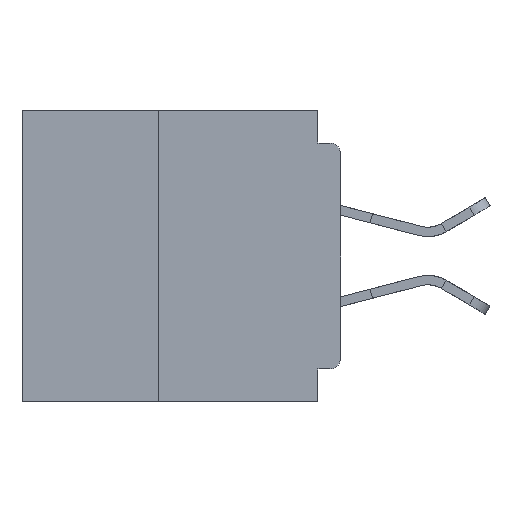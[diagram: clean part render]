
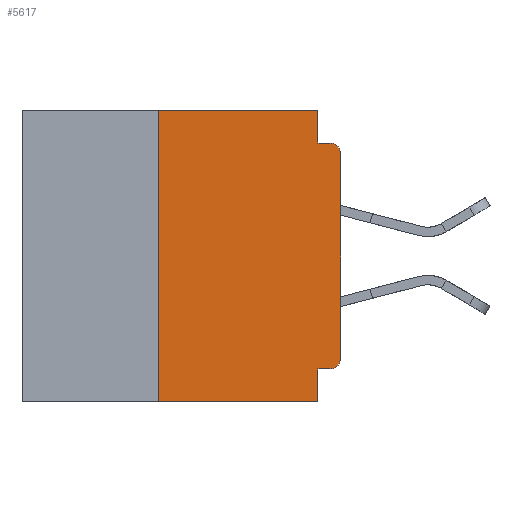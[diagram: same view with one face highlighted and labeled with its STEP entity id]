
A CAD part, left-side view. The second image highlights one B-rep face of the part: STEP entity #5617.
In plain terms, the highlighted planar face has unit normal (-1, 0, 0).
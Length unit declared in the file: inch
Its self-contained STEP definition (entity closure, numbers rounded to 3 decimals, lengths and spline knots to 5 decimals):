
#760 = EDGE_LOOP ( 'NONE', ( #19155, #7174, #18591, #26904, #25156, #31507, #24064, #19245, #5497, #3072 ) ) ;
#850 = DIRECTION ( 'NONE',  ( 0., -1., 0. ) ) ;
#874 = VECTOR ( 'NONE', #28364, 39.37008 ) ;
#1876 = CARTESIAN_POINT ( 'NONE',  ( 0., 0.031, -0.355 ) ) ;
#2531 = CIRCLE ( 'NONE', #13504, 0.015 ) ;
#3072 = ORIENTED_EDGE ( 'NONE', *, *, #12800, .T. ) ;
#3850 = LINE ( 'NONE', #40237, #29179 ) ;
#5197 = DIRECTION ( 'NONE',  ( -1., 0., 0. ) ) ;
#5497 = ORIENTED_EDGE ( 'NONE', *, *, #16973, .F. ) ;
#5546 = LINE ( 'NONE', #32542, #23152 ) ;
#5617 = ADVANCED_FACE ( 'NONE', ( #33555 ), #7293, .F. ) ;
#5638 = CARTESIAN_POINT ( 'NONE',  ( 0., 0., -0.34 ) ) ;
#6015 = VERTEX_POINT ( 'NONE', #8084 ) ;
#6121 = CARTESIAN_POINT ( 'NONE',  ( 0., 0.015, -0.34 ) ) ;
#6954 = CARTESIAN_POINT ( 'NONE',  ( 0., 0., 0. ) ) ;
#7174 = ORIENTED_EDGE ( 'NONE', *, *, #29271, .T. ) ;
#7293 = PLANE ( 'NONE',  #39121 ) ;
#8084 = CARTESIAN_POINT ( 'NONE',  ( 0., 0., -0.06 ) ) ;
#9132 = LINE ( 'NONE', #10199, #25701 ) ;
#9355 = CARTESIAN_POINT ( 'NONE',  ( 0., 0.031, -0.4 ) ) ;
#9437 = DIRECTION ( 'NONE',  ( 0., 0., -1. ) ) ;
#9480 = DIRECTION ( 'NONE',  ( 0., 0., -1. ) ) ;
#9642 = VERTEX_POINT ( 'NONE', #5638 ) ;
#10199 = CARTESIAN_POINT ( 'NONE',  ( 0., 0., -0.045 ) ) ;
#10797 = VERTEX_POINT ( 'NONE', #1876 ) ;
#11813 = VECTOR ( 'NONE', #39659, 39.37008 ) ;
#12800 = EDGE_CURVE ( 'NONE', #18607, #9642, #20574, .T. ) ;
#12972 = EDGE_CURVE ( 'NONE', #9642, #6015, #23135, .T. ) ;
#13504 = AXIS2_PLACEMENT_3D ( 'NONE', #25016, #5197, #28303 ) ;
#13541 = DIRECTION ( 'NONE',  ( 0., -1., 0. ) ) ;
#13967 = VECTOR ( 'NONE', #14955, 39.37008 ) ;
#14865 = VERTEX_POINT ( 'NONE', #29692 ) ;
#14955 = DIRECTION ( 'NONE',  ( 0., 1., 0. ) ) ;
#16574 = VERTEX_POINT ( 'NONE', #9355 ) ;
#16596 = CARTESIAN_POINT ( 'NONE',  ( 0., 0.031, -0.4 ) ) ;
#16973 = EDGE_CURVE ( 'NONE', #18607, #10797, #22765, .T. ) ;
#17788 = EDGE_CURVE ( 'NONE', #14865, #20665, #26785, .T. ) ;
#18015 = VECTOR ( 'NONE', #40280, 39.37008 ) ;
#18419 = CARTESIAN_POINT ( 'NONE',  ( 0., 0.437, -0.4 ) ) ;
#18591 = ORIENTED_EDGE ( 'NONE', *, *, #30137, .F. ) ;
#18607 = VERTEX_POINT ( 'NONE', #41528 ) ;
#19155 = ORIENTED_EDGE ( 'NONE', *, *, #12972, .T. ) ;
#19245 = ORIENTED_EDGE ( 'NONE', *, *, #34784, .F. ) ;
#20331 = EDGE_CURVE ( 'NONE', #20665, #31891, #3850, .T. ) ;
#20574 = CIRCLE ( 'NONE', #31055, 0.015 ) ;
#20590 = CARTESIAN_POINT ( 'NONE',  ( 0., 0.25, -0.4 ) ) ;
#20630 = LINE ( 'NONE', #16596, #11813 ) ;
#20636 = DIRECTION ( 'NONE',  ( 0., 0., -1. ) ) ;
#20665 = VERTEX_POINT ( 'NONE', #22701 ) ;
#22105 = VECTOR ( 'NONE', #26763, 39.37008 ) ;
#22701 = CARTESIAN_POINT ( 'NONE',  ( 0., 0.25, 0. ) ) ;
#22765 = LINE ( 'NONE', #28092, #13967 ) ;
#23135 = LINE ( 'NONE', #6954, #22105 ) ;
#23152 = VECTOR ( 'NONE', #9480, 39.37008 ) ;
#23533 = CARTESIAN_POINT ( 'NONE',  ( 0., 0.015, -0.045 ) ) ;
#24064 = ORIENTED_EDGE ( 'NONE', *, *, #25652, .T. ) ;
#25016 = CARTESIAN_POINT ( 'NONE',  ( 0., 0.015, -0.06 ) ) ;
#25156 = ORIENTED_EDGE ( 'NONE', *, *, #20331, .F. ) ;
#25652 = EDGE_CURVE ( 'NONE', #14865, #16574, #35983, .T. ) ;
#25701 = VECTOR ( 'NONE', #13541, 39.37008 ) ;
#26738 = CARTESIAN_POINT ( 'NONE',  ( 0., 0.031, -0.045 ) ) ;
#26763 = DIRECTION ( 'NONE',  ( 0., 0., 1. ) ) ;
#26785 = LINE ( 'NONE', #20590, #18015 ) ;
#26904 = ORIENTED_EDGE ( 'NONE', *, *, #35365, .F. ) ;
#28092 = CARTESIAN_POINT ( 'NONE',  ( 0., 0., -0.355 ) ) ;
#28303 = DIRECTION ( 'NONE',  ( 0., 0., -1. ) ) ;
#28364 = DIRECTION ( 'NONE',  ( 0., -1., 0. ) ) ;
#29179 = VECTOR ( 'NONE', #850, 39.37008 ) ;
#29206 = DIRECTION ( 'NONE',  ( -1., 0., 0. ) ) ;
#29271 = EDGE_CURVE ( 'NONE', #6015, #42023, #2531, .T. ) ;
#29692 = CARTESIAN_POINT ( 'NONE',  ( 0., 0.25, -0.4 ) ) ;
#30137 = EDGE_CURVE ( 'NONE', #39871, #42023, #9132, .T. ) ;
#30398 = CARTESIAN_POINT ( 'NONE',  ( 0., 0.437, 0. ) ) ;
#31055 = AXIS2_PLACEMENT_3D ( 'NONE', #6121, #29206, #9437 ) ;
#31507 = ORIENTED_EDGE ( 'NONE', *, *, #17788, .F. ) ;
#31891 = VERTEX_POINT ( 'NONE', #38903 ) ;
#32542 = CARTESIAN_POINT ( 'NONE',  ( 0., 0.031, 0. ) ) ;
#33555 = FACE_OUTER_BOUND ( 'NONE', #760, .T. ) ;
#34784 = EDGE_CURVE ( 'NONE', #10797, #16574, #20630, .T. ) ;
#35365 = EDGE_CURVE ( 'NONE', #31891, #39871, #5546, .T. ) ;
#35983 = LINE ( 'NONE', #18419, #874 ) ;
#38903 = CARTESIAN_POINT ( 'NONE',  ( 0., 0.031, 0. ) ) ;
#39121 = AXIS2_PLACEMENT_3D ( 'NONE', #30398, #40325, #20636 ) ;
#39659 = DIRECTION ( 'NONE',  ( 0., 0., -1. ) ) ;
#39871 = VERTEX_POINT ( 'NONE', #26738 ) ;
#40237 = CARTESIAN_POINT ( 'NONE',  ( 0., 0.437, 0. ) ) ;
#40280 = DIRECTION ( 'NONE',  ( 0., 0., 1. ) ) ;
#40325 = DIRECTION ( 'NONE',  ( 1., 0., 0. ) ) ;
#41528 = CARTESIAN_POINT ( 'NONE',  ( 0., 0.015, -0.355 ) ) ;
#42023 = VERTEX_POINT ( 'NONE', #23533 ) ;
